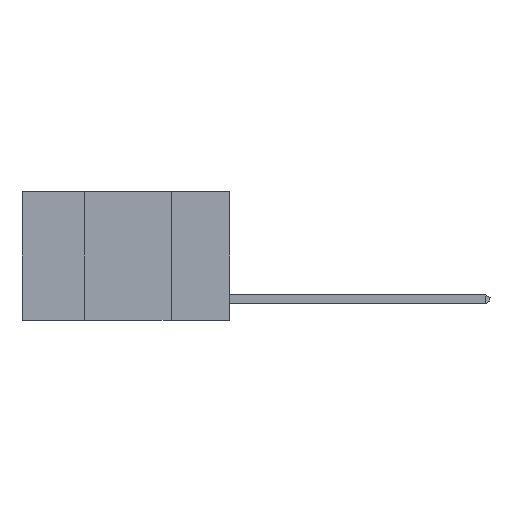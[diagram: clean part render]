
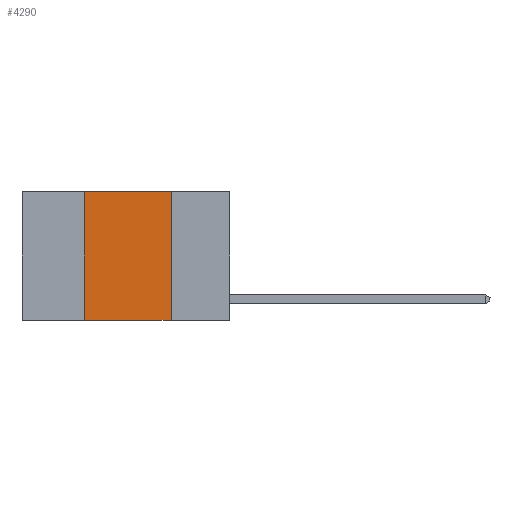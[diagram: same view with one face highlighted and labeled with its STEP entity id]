
A CAD part, left-side view. The second image highlights one B-rep face of the part: STEP entity #4290.
In plain terms, the highlighted planar face has unit normal (-1, 0, 0).
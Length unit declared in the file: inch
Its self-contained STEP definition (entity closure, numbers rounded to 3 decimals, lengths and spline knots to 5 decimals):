
#52 = EDGE_CURVE ( 'NONE', #19517, #3703, #5273, .T. ) ;
#608 = DIRECTION ( 'NONE',  ( 0., -1., 0. ) ) ;
#630 = CARTESIAN_POINT ( 'NONE',  ( 0., 0.42, -0.37 ) ) ;
#1077 = CARTESIAN_POINT ( 'NONE',  ( 0., 0.42, 0. ) ) ;
#1144 = VECTOR ( 'NONE', #608, 39.37008 ) ;
#1499 = DIRECTION ( 'NONE',  ( 0., -1., 0. ) ) ;
#2236 = FACE_OUTER_BOUND ( 'NONE', #13683, .T. ) ;
#2289 = EDGE_CURVE ( 'NONE', #15029, #19517, #14014, .T. ) ;
#3390 = VECTOR ( 'NONE', #15765, 39.37008 ) ;
#3703 = VERTEX_POINT ( 'NONE', #15566 ) ;
#4290 = ADVANCED_FACE ( 'NONE', ( #2236 ), #16791, .F. ) ;
#4350 = DIRECTION ( 'NONE',  ( 1., 0., 0. ) ) ;
#4459 = CARTESIAN_POINT ( 'NONE',  ( 0., 0.6, 0. ) ) ;
#5273 = LINE ( 'NONE', #19391, #7463 ) ;
#7463 = VECTOR ( 'NONE', #1499, 39.37008 ) ;
#8044 = LINE ( 'NONE', #15174, #18133 ) ;
#8674 = AXIS2_PLACEMENT_3D ( 'NONE', #4459, #4350, #21894 ) ;
#10347 = EDGE_CURVE ( 'NONE', #15029, #16132, #13075, .T. ) ;
#10660 = CARTESIAN_POINT ( 'NONE',  ( 0., 0.17, -0.37 ) ) ;
#11180 = ORIENTED_EDGE ( 'NONE', *, *, #52, .F. ) ;
#12530 = CARTESIAN_POINT ( 'NONE',  ( 0., 0.42, 0. ) ) ;
#13075 = LINE ( 'NONE', #20266, #1144 ) ;
#13166 = ORIENTED_EDGE ( 'NONE', *, *, #13847, .F. ) ;
#13413 = DIRECTION ( 'NONE',  ( 0., 0., -1. ) ) ;
#13683 = EDGE_LOOP ( 'NONE', ( #13166, #11180, #19654, #17397 ) ) ;
#13847 = EDGE_CURVE ( 'NONE', #3703, #16132, #8044, .T. ) ;
#14014 = LINE ( 'NONE', #1077, #3390 ) ;
#15029 = VERTEX_POINT ( 'NONE', #630 ) ;
#15174 = CARTESIAN_POINT ( 'NONE',  ( 0., 0.17, 0. ) ) ;
#15566 = CARTESIAN_POINT ( 'NONE',  ( 0., 0.17, 0. ) ) ;
#15765 = DIRECTION ( 'NONE',  ( 0., 0., 1. ) ) ;
#16132 = VERTEX_POINT ( 'NONE', #10660 ) ;
#16791 = PLANE ( 'NONE',  #8674 ) ;
#17397 = ORIENTED_EDGE ( 'NONE', *, *, #10347, .T. ) ;
#18133 = VECTOR ( 'NONE', #13413, 39.37008 ) ;
#19391 = CARTESIAN_POINT ( 'NONE',  ( 0., 0.6, 0. ) ) ;
#19517 = VERTEX_POINT ( 'NONE', #12530 ) ;
#19654 = ORIENTED_EDGE ( 'NONE', *, *, #2289, .F. ) ;
#20266 = CARTESIAN_POINT ( 'NONE',  ( 0., 0.6, -0.37 ) ) ;
#21894 = DIRECTION ( 'NONE',  ( 0., 0., -1. ) ) ;
